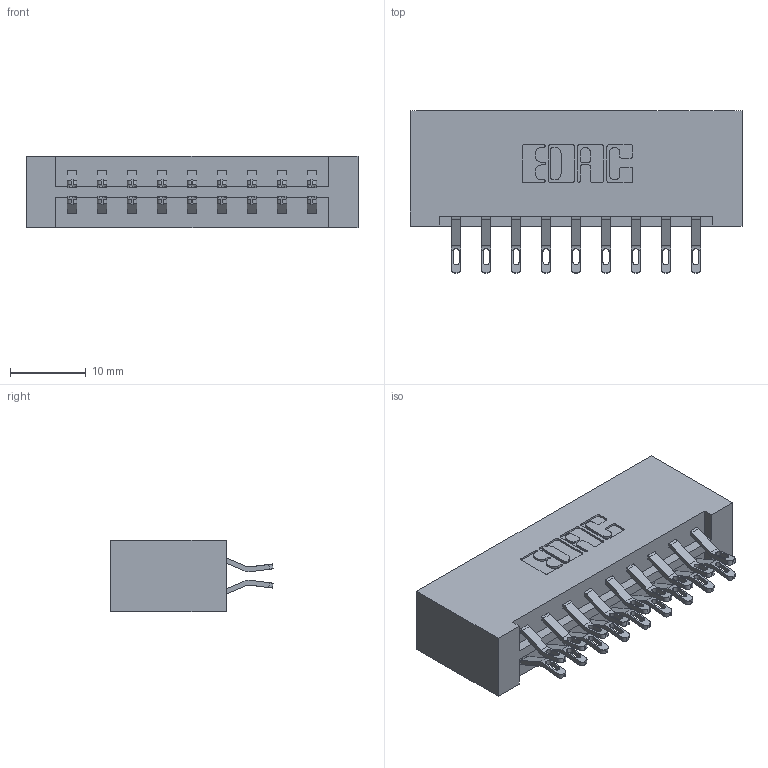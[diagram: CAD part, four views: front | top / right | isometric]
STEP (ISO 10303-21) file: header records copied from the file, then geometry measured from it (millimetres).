
FILE_DESCRIPTION (( 'STEP AP203' ), '1' );
FILE_NAME ('833-018-555-201.STEP', '2020-05-31T22:53:46', ( '' ), ( '' ), 'SwSTEP 2.0', 'SolidWorks 2020', '' );
FILE_SCHEMA (( 'CONFIG_CONTROL_DESIGN' ));
Length unit declared in the file: inch
Products named in the file (3): 833 Part_Lugless; 833-018-555-201; 345-292-001_555 Tail
Assembly tree (19 placements, depth 2):
  833-018-555-201
    833 Part_Lugless
    345-292-001_555 Tail  x18
Bounding box: 43.92 x 21.47 x 9.4 mm (x, y, z)
Volume: 4859.5 mm3; surface area: 5610.1 mm2
Topology: 19 solids, 19 shells, 1150 faces, 3581 edges, 2386 vertices
Faces by surface type: plane 678, cylinder 472
Entity records: 10107 total; most frequent: CARTESIAN_POINT 1748, ORIENTED_EDGE 1654, DIRECTION 1515, EDGE_CURVE 827, LINE 687, VECTOR 687, VERTEX_POINT 550, AXIS2_PLACEMENT_3D 414
